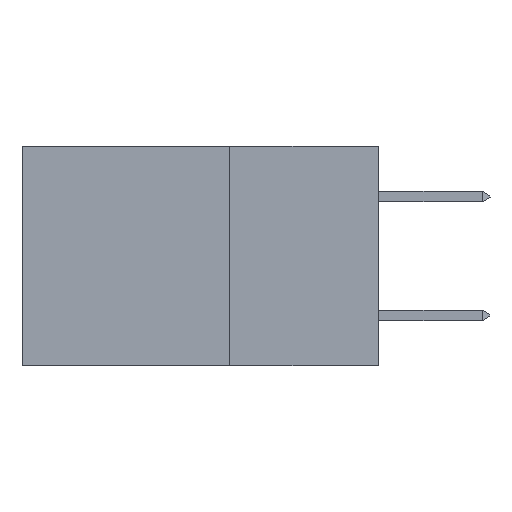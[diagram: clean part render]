
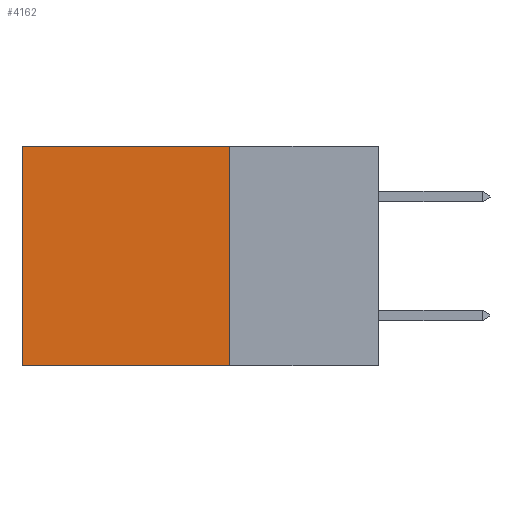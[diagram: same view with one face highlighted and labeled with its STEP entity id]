
A CAD part, left-side view. The second image highlights one B-rep face of the part: STEP entity #4162.
In plain terms, the highlighted planar face has unit normal (-1, 0, 0).
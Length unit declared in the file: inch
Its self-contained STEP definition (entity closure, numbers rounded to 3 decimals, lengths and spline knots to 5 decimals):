
#278 = EDGE_CURVE ( 'NONE', #26966, #29019, #7312, .T. ) ;
#970 = CARTESIAN_POINT ( 'NONE',  ( 0.298, 0.25, -0.37 ) ) ;
#1406 = LINE ( 'NONE', #7455, #18098 ) ;
#3240 = ORIENTED_EDGE ( 'NONE', *, *, #22576, .T. ) ;
#3600 = DIRECTION ( 'NONE',  ( 0., 1., 0. ) ) ;
#4162 = ADVANCED_FACE ( 'NONE', ( #23948 ), #8995, .F. ) ;
#5012 = ORIENTED_EDGE ( 'NONE', *, *, #25139, .F. ) ;
#5519 = CARTESIAN_POINT ( 'NONE',  ( 0.298, 0.25, 0. ) ) ;
#6818 = DIRECTION ( 'NONE',  ( 1., 0., 0. ) ) ;
#7312 = LINE ( 'NONE', #28244, #27211 ) ;
#7455 = CARTESIAN_POINT ( 'NONE',  ( 0.298, 0.6, 0. ) ) ;
#7669 = LINE ( 'NONE', #970, #10782 ) ;
#7726 = VERTEX_POINT ( 'NONE', #18930 ) ;
#8995 = PLANE ( 'NONE',  #15640 ) ;
#10560 = ORIENTED_EDGE ( 'NONE', *, *, #278, .F. ) ;
#10782 = VECTOR ( 'NONE', #21313, 39.37008 ) ;
#14577 = DIRECTION ( 'NONE',  ( 0., 0., -1. ) ) ;
#15640 = AXIS2_PLACEMENT_3D ( 'NONE', #20399, #6818, #29412 ) ;
#16741 = EDGE_LOOP ( 'NONE', ( #3240, #5012, #10560, #24224 ) ) ;
#17733 = CARTESIAN_POINT ( 'NONE',  ( 0.298, 0.25, -0.37 ) ) ;
#18098 = VECTOR ( 'NONE', #14577, 39.37008 ) ;
#18294 = CARTESIAN_POINT ( 'NONE',  ( 0.298, 0.6, 0. ) ) ;
#18491 = CARTESIAN_POINT ( 'NONE',  ( 0.298, 0.25, 0. ) ) ;
#18930 = CARTESIAN_POINT ( 'NONE',  ( 0.298, 0.6, -0.37 ) ) ;
#19227 = VECTOR ( 'NONE', #3600, 39.37008 ) ;
#20399 = CARTESIAN_POINT ( 'NONE',  ( 0.298, 0.25, 0. ) ) ;
#21313 = DIRECTION ( 'NONE',  ( 0., 1., 0. ) ) ;
#21446 = DIRECTION ( 'NONE',  ( 0., 0., -1. ) ) ;
#21632 = VERTEX_POINT ( 'NONE', #18294 ) ;
#22426 = LINE ( 'NONE', #5519, #19227 ) ;
#22576 = EDGE_CURVE ( 'NONE', #21632, #7726, #1406, .T. ) ;
#23948 = FACE_OUTER_BOUND ( 'NONE', #16741, .T. ) ;
#24224 = ORIENTED_EDGE ( 'NONE', *, *, #27161, .T. ) ;
#25139 = EDGE_CURVE ( 'NONE', #29019, #7726, #7669, .T. ) ;
#26966 = VERTEX_POINT ( 'NONE', #18491 ) ;
#27161 = EDGE_CURVE ( 'NONE', #26966, #21632, #22426, .T. ) ;
#27211 = VECTOR ( 'NONE', #21446, 39.37008 ) ;
#28244 = CARTESIAN_POINT ( 'NONE',  ( 0.298, 0.25, 0. ) ) ;
#29019 = VERTEX_POINT ( 'NONE', #17733 ) ;
#29412 = DIRECTION ( 'NONE',  ( 0., 0., -1. ) ) ;
